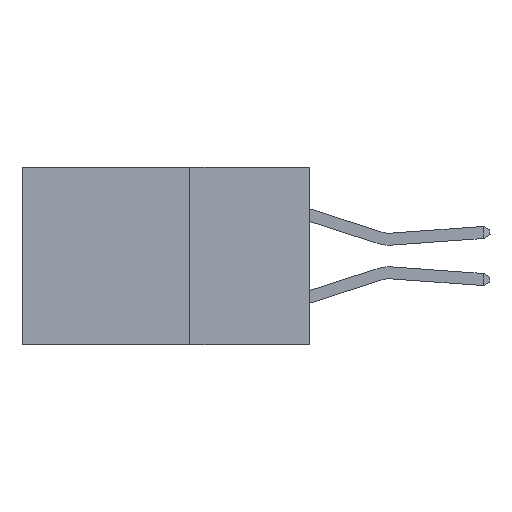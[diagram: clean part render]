
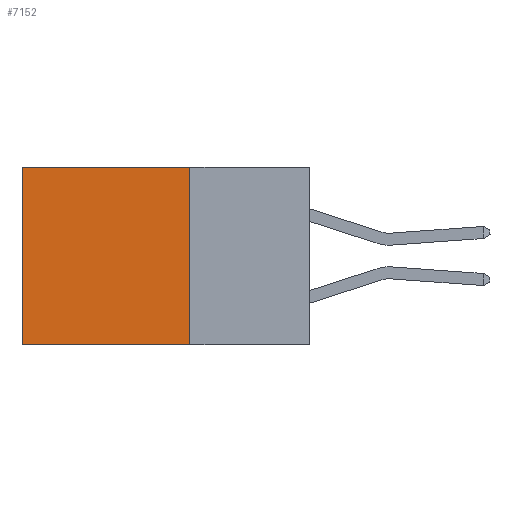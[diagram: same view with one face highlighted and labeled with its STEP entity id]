
A CAD part, left-side view. The second image highlights one B-rep face of the part: STEP entity #7152.
In plain terms, the highlighted planar face has unit normal (-1, 0, 0).
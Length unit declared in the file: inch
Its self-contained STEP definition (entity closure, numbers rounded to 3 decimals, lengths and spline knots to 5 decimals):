
#121 = VERTEX_POINT ( 'NONE', #11908 ) ;
#743 = DIRECTION ( 'NONE',  ( 0., 0., -1. ) ) ;
#1806 = DIRECTION ( 'NONE',  ( 0., 1., 0. ) ) ;
#2005 = VERTEX_POINT ( 'NONE', #7427 ) ;
#2061 = DIRECTION ( 'NONE',  ( 0., 0., -1. ) ) ;
#2359 = VERTEX_POINT ( 'NONE', #3087 ) ;
#2390 = EDGE_CURVE ( 'NONE', #2359, #10847, #9407, .T. ) ;
#2640 = ORIENTED_EDGE ( 'NONE', *, *, #4274, .F. ) ;
#2878 = AXIS2_PLACEMENT_3D ( 'NONE', #5556, #8102, #13225 ) ;
#3087 = CARTESIAN_POINT ( 'NONE',  ( 0.2615, 0.25, 0. ) ) ;
#3641 = CARTESIAN_POINT ( 'NONE',  ( 0.2615, 0.25, -0.37 ) ) ;
#4274 = EDGE_CURVE ( 'NONE', #2359, #2005, #13702, .T. ) ;
#4369 = CARTESIAN_POINT ( 'NONE',  ( 0.2615, 0.6, 0. ) ) ;
#4659 = DIRECTION ( 'NONE',  ( 0., 1., 0. ) ) ;
#4692 = ORIENTED_EDGE ( 'NONE', *, *, #2390, .T. ) ;
#5556 = CARTESIAN_POINT ( 'NONE',  ( 0.2615, 0.25, -0.37 ) ) ;
#6486 = FACE_OUTER_BOUND ( 'NONE', #9184, .T. ) ;
#7152 = ADVANCED_FACE ( 'NONE', ( #6486 ), #7839, .F. ) ;
#7229 = CARTESIAN_POINT ( 'NONE',  ( 0.2615, 0.25, -0.37 ) ) ;
#7427 = CARTESIAN_POINT ( 'NONE',  ( 0.2615, 0.25, -0.37 ) ) ;
#7839 = PLANE ( 'NONE',  #2878 ) ;
#7897 = ORIENTED_EDGE ( 'NONE', *, *, #13838, .T. ) ;
#8102 = DIRECTION ( 'NONE',  ( 1., 0., 0. ) ) ;
#8286 = VECTOR ( 'NONE', #1806, 39.37008 ) ;
#8524 = LINE ( 'NONE', #13723, #10854 ) ;
#9184 = EDGE_LOOP ( 'NONE', ( #7897, #16824, #2640, #4692 ) ) ;
#9407 = LINE ( 'NONE', #13473, #8286 ) ;
#10412 = VECTOR ( 'NONE', #4659, 39.37008 ) ;
#10847 = VERTEX_POINT ( 'NONE', #4369 ) ;
#10854 = VECTOR ( 'NONE', #2061, 39.37008 ) ;
#11908 = CARTESIAN_POINT ( 'NONE',  ( 0.2615, 0.6, -0.37 ) ) ;
#12509 = LINE ( 'NONE', #3641, #10412 ) ;
#13225 = DIRECTION ( 'NONE',  ( 0., 0., -1. ) ) ;
#13473 = CARTESIAN_POINT ( 'NONE',  ( 0.2615, 0.25, 0. ) ) ;
#13702 = LINE ( 'NONE', #7229, #14375 ) ;
#13723 = CARTESIAN_POINT ( 'NONE',  ( 0.2615, 0.6, -0.37 ) ) ;
#13838 = EDGE_CURVE ( 'NONE', #10847, #121, #8524, .T. ) ;
#14375 = VECTOR ( 'NONE', #743, 39.37008 ) ;
#14426 = EDGE_CURVE ( 'NONE', #2005, #121, #12509, .T. ) ;
#16824 = ORIENTED_EDGE ( 'NONE', *, *, #14426, .F. ) ;
